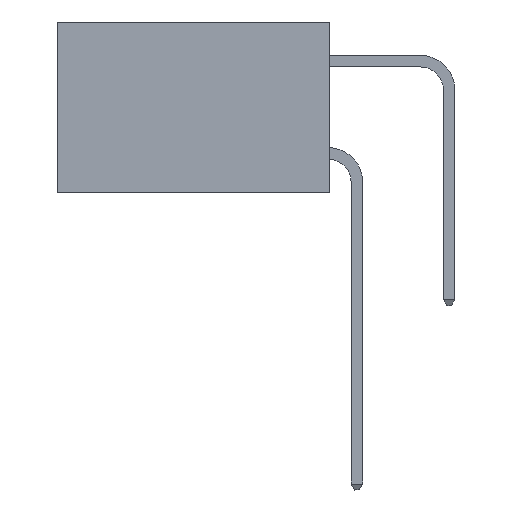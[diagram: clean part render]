
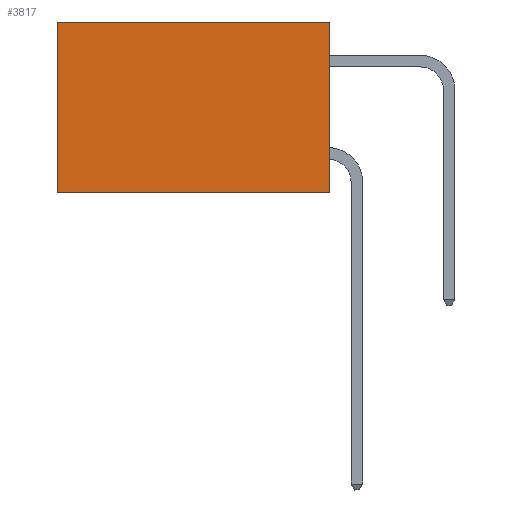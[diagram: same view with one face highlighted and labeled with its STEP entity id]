
A CAD part, left-side view. The second image highlights one B-rep face of the part: STEP entity #3817.
In plain terms, the highlighted planar face has unit normal (-1, 0, 0).
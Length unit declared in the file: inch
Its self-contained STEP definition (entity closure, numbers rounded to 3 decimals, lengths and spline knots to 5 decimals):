
#64 = ORIENTED_EDGE ( 'NONE', *, *, #13188, .F. ) ;
#221 = LINE ( 'NONE', #11087, #5730 ) ;
#534 = DIRECTION ( 'NONE',  ( 0., 0., -1. ) ) ;
#854 = DIRECTION ( 'NONE',  ( 1., 0., 0. ) ) ;
#1013 = CARTESIAN_POINT ( 'NONE',  ( 0.277, 0., 0. ) ) ;
#1041 = CARTESIAN_POINT ( 'NONE',  ( 0.277, 0., -0.37 ) ) ;
#1792 = ORIENTED_EDGE ( 'NONE', *, *, #4742, .T. ) ;
#1923 = CARTESIAN_POINT ( 'NONE',  ( 0.277, 0.59, -0.37 ) ) ;
#1930 = LINE ( 'NONE', #9042, #7738 ) ;
#1950 = ORIENTED_EDGE ( 'NONE', *, *, #3176, .T. ) ;
#2020 = PLANE ( 'NONE',  #5631 ) ;
#2114 = CARTESIAN_POINT ( 'NONE',  ( 0.277, 0.59, -0.37 ) ) ;
#2224 = VECTOR ( 'NONE', #8011, 39.37008 ) ;
#2311 = DIRECTION ( 'NONE',  ( 0., 0., -1. ) ) ;
#2478 = DIRECTION ( 'NONE',  ( 0., 1., 0. ) ) ;
#3176 = EDGE_CURVE ( 'NONE', #8822, #8714, #12489, .T. ) ;
#3817 = ADVANCED_FACE ( 'NONE', ( #9461 ), #2020, .F. ) ;
#3833 = VECTOR ( 'NONE', #11498, 39.37008 ) ;
#4349 = EDGE_LOOP ( 'NONE', ( #1950, #64, #4392, #1792 ) ) ;
#4392 = ORIENTED_EDGE ( 'NONE', *, *, #12349, .F. ) ;
#4742 = EDGE_CURVE ( 'NONE', #8851, #8822, #13742, .T. ) ;
#5631 = AXIS2_PLACEMENT_3D ( 'NONE', #1041, #854, #534 ) ;
#5730 = VECTOR ( 'NONE', #2311, 39.37008 ) ;
#7738 = VECTOR ( 'NONE', #2478, 39.37008 ) ;
#8011 = DIRECTION ( 'NONE',  ( 0., 1., 0. ) ) ;
#8068 = CARTESIAN_POINT ( 'NONE',  ( 0.277, 0., 0. ) ) ;
#8714 = VERTEX_POINT ( 'NONE', #1923 ) ;
#8822 = VERTEX_POINT ( 'NONE', #11966 ) ;
#8851 = VERTEX_POINT ( 'NONE', #1013 ) ;
#9042 = CARTESIAN_POINT ( 'NONE',  ( 0.277, 0., -0.37 ) ) ;
#9461 = FACE_OUTER_BOUND ( 'NONE', #4349, .T. ) ;
#11087 = CARTESIAN_POINT ( 'NONE',  ( 0.277, 0., -0.37 ) ) ;
#11498 = DIRECTION ( 'NONE',  ( 0., 0., -1. ) ) ;
#11966 = CARTESIAN_POINT ( 'NONE',  ( 0.277, 0.59, 0. ) ) ;
#12249 = VERTEX_POINT ( 'NONE', #13861 ) ;
#12349 = EDGE_CURVE ( 'NONE', #8851, #12249, #221, .T. ) ;
#12489 = LINE ( 'NONE', #2114, #3833 ) ;
#13188 = EDGE_CURVE ( 'NONE', #12249, #8714, #1930, .T. ) ;
#13742 = LINE ( 'NONE', #8068, #2224 ) ;
#13861 = CARTESIAN_POINT ( 'NONE',  ( 0.277, 0., -0.37 ) ) ;
